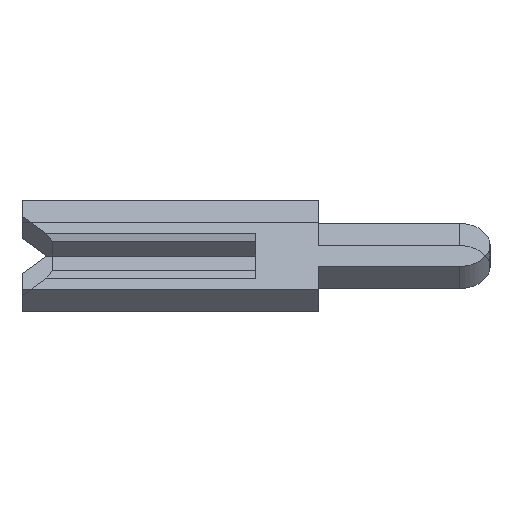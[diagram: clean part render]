
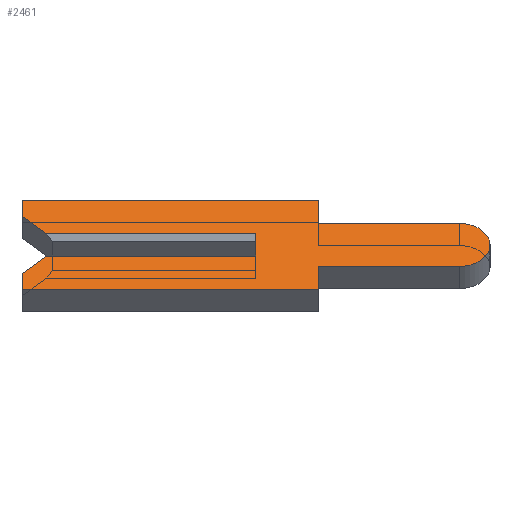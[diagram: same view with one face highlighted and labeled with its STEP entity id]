
A CAD part, left-side view. The second image highlights one B-rep face of the part: STEP entity #2461.
In plain terms, the highlighted face is planar.
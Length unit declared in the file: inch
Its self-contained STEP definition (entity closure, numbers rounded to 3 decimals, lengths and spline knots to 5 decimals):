
#58 = CARTESIAN_POINT ( 'NONE',  ( -0.01, 0.134, 0.01 ) ) ;
#107 = VECTOR ( 'NONE', #3447, 39.37008 ) ;
#141 = DIRECTION ( 'NONE',  ( 1., 0., 0. ) ) ;
#152 = VECTOR ( 'NONE', #665, 39.37008 ) ;
#166 = CARTESIAN_POINT ( 'NONE',  ( -0.01, 0.15, 0.04 ) ) ;
#196 = CARTESIAN_POINT ( 'NONE',  ( -0.01, -0.04, 0.04 ) ) ;
#232 = CARTESIAN_POINT ( 'NONE',  ( -0.01, 0.1305, 0.0065 ) ) ;
#246 = EDGE_CURVE ( 'NONE', #1155, #625, #2005, .T. ) ;
#277 = CARTESIAN_POINT ( 'NONE',  ( -0.01, -0.04, -0.04 ) ) ;
#285 = CARTESIAN_POINT ( 'NONE',  ( -0.01, -0.1305, 0. ) ) ;
#288 = EDGE_LOOP ( 'NONE', ( #2585, #559, #1931, #608, #2971, #2772, #2966, #3090, #3559, #2546, #3043, #3548, #3137, #441 ) ) ;
#347 = CARTESIAN_POINT ( 'NONE',  ( -0.01, 0.15, 0.04 ) ) ;
#351 = EDGE_CURVE ( 'NONE', #2075, #1006, #2278, .T. ) ;
#366 = CARTESIAN_POINT ( 'NONE',  ( -0.01, 0.15, 0.026 ) ) ;
#377 = AXIS2_PLACEMENT_3D ( 'NONE', #285, #3104, #556 ) ;
#441 = ORIENTED_EDGE ( 'NONE', *, *, #246, .F. ) ;
#442 = EDGE_CURVE ( 'NONE', #2650, #2375, #3222, .T. ) ;
#449 = FACE_OUTER_BOUND ( 'NONE', #288, .T. ) ;
#497 = VECTOR ( 'NONE', #2241, 39.37008 ) ;
#556 = DIRECTION ( 'NONE',  ( 0., 0., -1. ) ) ;
#559 = ORIENTED_EDGE ( 'NONE', *, *, #351, .F. ) ;
#578 = CARTESIAN_POINT ( 'NONE',  ( -0.01, -0.04, 0.0195 ) ) ;
#594 = DIRECTION ( 'NONE',  ( 0., 1., 0. ) ) ;
#605 = VECTOR ( 'NONE', #3147, 39.37008 ) ;
#608 = ORIENTED_EDGE ( 'NONE', *, *, #2919, .F. ) ;
#615 = DIRECTION ( 'NONE',  ( 0., -1., 0. ) ) ;
#625 = VERTEX_POINT ( 'NONE', #1739 ) ;
#659 = VERTEX_POINT ( 'NONE', #277 ) ;
#665 = DIRECTION ( 'NONE',  ( 0., -1., 0. ) ) ;
#700 = VERTEX_POINT ( 'NONE', #1437 ) ;
#757 = CARTESIAN_POINT ( 'NONE',  ( -0.01, -0.04, -0.0195 ) ) ;
#759 = VECTOR ( 'NONE', #2761, 39.37008 ) ;
#804 = CARTESIAN_POINT ( 'NONE',  ( -0.01, 0.134, -0.01 ) ) ;
#827 = CARTESIAN_POINT ( 'NONE',  ( -0.01, 0.1305, -0.0065 ) ) ;
#945 = LINE ( 'NONE', #578, #3312 ) ;
#993 = VECTOR ( 'NONE', #594, 39.37008 ) ;
#1006 = VERTEX_POINT ( 'NONE', #2529 ) ;
#1013 = CARTESIAN_POINT ( 'NONE',  ( -0.01, -0.1305, 0. ) ) ;
#1029 = DIRECTION ( 'NONE',  ( 0., 0., -1. ) ) ;
#1109 = CARTESIAN_POINT ( 'NONE',  ( -0.01, 0.15, -0.04 ) ) ;
#1114 = VECTOR ( 'NONE', #1029, 39.37008 ) ;
#1142 = VERTEX_POINT ( 'NONE', #2064 ) ;
#1155 = VERTEX_POINT ( 'NONE', #58 ) ;
#1291 = EDGE_CURVE ( 'NONE', #2232, #659, #3451, .T. ) ;
#1321 = LINE ( 'NONE', #347, #152 ) ;
#1329 = EDGE_CURVE ( 'NONE', #2375, #2232, #2113, .T. ) ;
#1339 = CARTESIAN_POINT ( 'NONE',  ( -0.01, -0.1305, -0.0195 ) ) ;
#1400 = DIRECTION ( 'NONE',  ( 0., 0.707, 0.707 ) ) ;
#1421 = LINE ( 'NONE', #3419, #759 ) ;
#1437 = CARTESIAN_POINT ( 'NONE',  ( -0.01, -0.04, 0.0195 ) ) ;
#1439 = DIRECTION ( 'NONE',  ( 0., -1., 0. ) ) ;
#1487 = DIRECTION ( 'NONE',  ( 0., 1., 0. ) ) ;
#1583 = DIRECTION ( 'NONE',  ( 0., 0., -1. ) ) ;
#1584 = EDGE_CURVE ( 'NONE', #2768, #2075, #3236, .T. ) ;
#1620 = VECTOR ( 'NONE', #2818, 39.37008 ) ;
#1626 = EDGE_CURVE ( 'NONE', #625, #2020, #2063, .T. ) ;
#1662 = VERTEX_POINT ( 'NONE', #1757 ) ;
#1692 = LINE ( 'NONE', #1109, #993 ) ;
#1739 = CARTESIAN_POINT ( 'NONE',  ( -0.01, 0.15, 0.026 ) ) ;
#1757 = CARTESIAN_POINT ( 'NONE',  ( -0.01, -0.04, 0.04 ) ) ;
#1789 = CARTESIAN_POINT ( 'NONE',  ( -0.01, -0.1305, -0.01 ) ) ;
#1802 = LINE ( 'NONE', #2282, #605 ) ;
#1885 = CARTESIAN_POINT ( 'NONE',  ( -0.01, 0., -0.01 ) ) ;
#1912 = CARTESIAN_POINT ( 'NONE',  ( -0.01, 0., 0.0065 ) ) ;
#1931 = ORIENTED_EDGE ( 'NONE', *, *, #1584, .F. ) ;
#2004 = EDGE_CURVE ( 'NONE', #2020, #1662, #1321, .T. ) ;
#2005 = LINE ( 'NONE', #232, #2365 ) ;
#2020 = VERTEX_POINT ( 'NONE', #166 ) ;
#2063 = LINE ( 'NONE', #366, #2495 ) ;
#2064 = CARTESIAN_POINT ( 'NONE',  ( -0.01, 0.15, -0.026 ) ) ;
#2075 = VERTEX_POINT ( 'NONE', #1885 ) ;
#2113 = LINE ( 'NONE', #2908, #2688 ) ;
#2148 = EDGE_CURVE ( 'NONE', #1662, #700, #3426, .T. ) ;
#2232 = VERTEX_POINT ( 'NONE', #757 ) ;
#2241 = DIRECTION ( 'NONE',  ( 0., -0.707, 0.707 ) ) ;
#2278 = LINE ( 'NONE', #1912, #107 ) ;
#2282 = CARTESIAN_POINT ( 'NONE',  ( -0.01, 0.15, 0.01 ) ) ;
#2331 = VERTEX_POINT ( 'NONE', #3567 ) ;
#2365 = VECTOR ( 'NONE', #1400, 39.37008 ) ;
#2375 = VERTEX_POINT ( 'NONE', #1339 ) ;
#2400 = LINE ( 'NONE', #827, #497 ) ;
#2461 = ADVANCED_FACE ( 'NONE', ( #449 ), #2714, .F. ) ;
#2495 = VECTOR ( 'NONE', #3194, 39.37008 ) ;
#2529 = CARTESIAN_POINT ( 'NONE',  ( -0.01, 0., 0.01 ) ) ;
#2532 = CARTESIAN_POINT ( 'NONE',  ( -0.01, -0.04, -0.04 ) ) ;
#2546 = ORIENTED_EDGE ( 'NONE', *, *, #2992, .F. ) ;
#2585 = ORIENTED_EDGE ( 'NONE', *, *, #3425, .T. ) ;
#2642 = EDGE_CURVE ( 'NONE', #2331, #1142, #1421, .T. ) ;
#2650 = VERTEX_POINT ( 'NONE', #3092 ) ;
#2656 = VECTOR ( 'NONE', #615, 39.37008 ) ;
#2688 = VECTOR ( 'NONE', #1487, 39.37008 ) ;
#2714 = PLANE ( 'NONE',  #2849 ) ;
#2761 = DIRECTION ( 'NONE',  ( 0., 0., 1. ) ) ;
#2768 = VERTEX_POINT ( 'NONE', #804 ) ;
#2772 = ORIENTED_EDGE ( 'NONE', *, *, #2968, .F. ) ;
#2818 = DIRECTION ( 'NONE',  ( 0., 0., -1. ) ) ;
#2849 = AXIS2_PLACEMENT_3D ( 'NONE', #1013, #141, #1583 ) ;
#2908 = CARTESIAN_POINT ( 'NONE',  ( -0.01, -0.04, -0.0195 ) ) ;
#2919 = EDGE_CURVE ( 'NONE', #1142, #2768, #2400, .T. ) ;
#2966 = ORIENTED_EDGE ( 'NONE', *, *, #1291, .F. ) ;
#2968 = EDGE_CURVE ( 'NONE', #659, #2331, #1692, .T. ) ;
#2971 = ORIENTED_EDGE ( 'NONE', *, *, #2642, .F. ) ;
#2992 = EDGE_CURVE ( 'NONE', #700, #2650, #945, .T. ) ;
#3043 = ORIENTED_EDGE ( 'NONE', *, *, #2148, .F. ) ;
#3090 = ORIENTED_EDGE ( 'NONE', *, *, #1329, .F. ) ;
#3092 = CARTESIAN_POINT ( 'NONE',  ( -0.01, -0.1305, 0.0195 ) ) ;
#3104 = DIRECTION ( 'NONE',  ( 1., 0., 0. ) ) ;
#3137 = ORIENTED_EDGE ( 'NONE', *, *, #1626, .F. ) ;
#3147 = DIRECTION ( 'NONE',  ( 0., -1., 0. ) ) ;
#3194 = DIRECTION ( 'NONE',  ( 0., 0., 1. ) ) ;
#3222 = CIRCLE ( 'NONE', #377, 0.0195 ) ;
#3236 = LINE ( 'NONE', #1789, #2656 ) ;
#3312 = VECTOR ( 'NONE', #1439, 39.37008 ) ;
#3419 = CARTESIAN_POINT ( 'NONE',  ( -0.01, 0.15, -0.026 ) ) ;
#3425 = EDGE_CURVE ( 'NONE', #1155, #1006, #1802, .T. ) ;
#3426 = LINE ( 'NONE', #196, #1114 ) ;
#3447 = DIRECTION ( 'NONE',  ( 0., 0., 1. ) ) ;
#3451 = LINE ( 'NONE', #2532, #1620 ) ;
#3548 = ORIENTED_EDGE ( 'NONE', *, *, #2004, .F. ) ;
#3559 = ORIENTED_EDGE ( 'NONE', *, *, #442, .F. ) ;
#3567 = CARTESIAN_POINT ( 'NONE',  ( -0.01, 0.15, -0.04 ) ) ;
